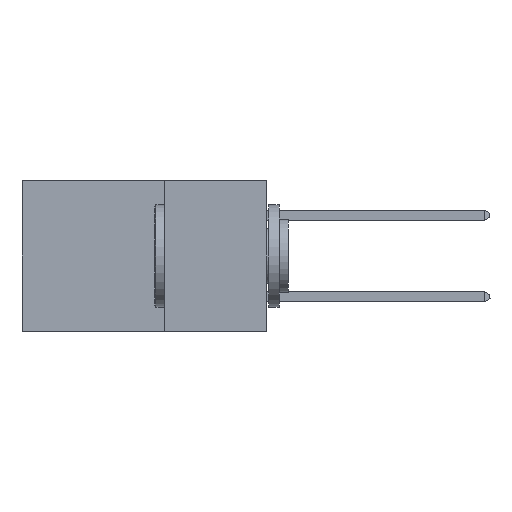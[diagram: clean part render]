
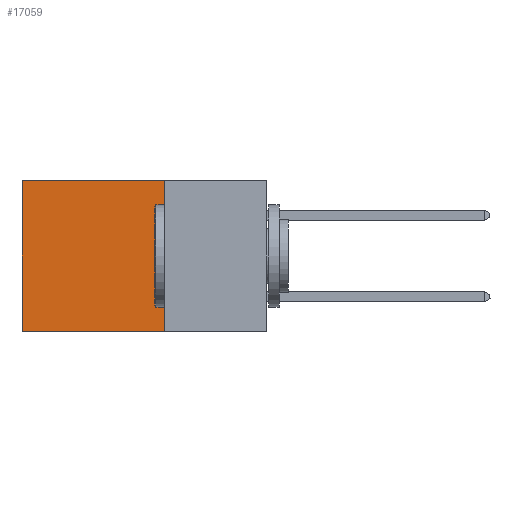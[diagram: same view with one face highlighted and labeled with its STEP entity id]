
A CAD part, left-side view. The second image highlights one B-rep face of the part: STEP entity #17059.
In plain terms, the highlighted planar face has unit normal (-1, 0, 0).
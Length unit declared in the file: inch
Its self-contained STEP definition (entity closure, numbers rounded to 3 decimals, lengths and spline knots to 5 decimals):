
#346 = VECTOR ( 'NONE', #17457, 39.37008 ) ;
#575 = DIRECTION ( 'NONE',  ( 0., 0., -1. ) ) ;
#2015 = LINE ( 'NONE', #3755, #9354 ) ;
#2084 = DIRECTION ( 'NONE',  ( 0., 1., 0. ) ) ;
#2139 = CARTESIAN_POINT ( 'NONE',  ( 0.2875, 0.6, 0. ) ) ;
#2925 = CARTESIAN_POINT ( 'NONE',  ( 0.2875, 0.6, 0. ) ) ;
#3717 = CARTESIAN_POINT ( 'NONE',  ( 0.2875, 0.25, 0. ) ) ;
#3755 = CARTESIAN_POINT ( 'NONE',  ( 0.2875, 0.25, 0. ) ) ;
#3989 = CARTESIAN_POINT ( 'NONE',  ( 0.2875, 0.25, -0.37 ) ) ;
#5107 = VERTEX_POINT ( 'NONE', #3989 ) ;
#5269 = CARTESIAN_POINT ( 'NONE',  ( 0.2875, 0.25, -0.37 ) ) ;
#5874 = ORIENTED_EDGE ( 'NONE', *, *, #10769, .F. ) ;
#6649 = ORIENTED_EDGE ( 'NONE', *, *, #21062, .T. ) ;
#6776 = AXIS2_PLACEMENT_3D ( 'NONE', #18778, #16770, #575 ) ;
#7679 = CARTESIAN_POINT ( 'NONE',  ( 0.2875, 0.25, 0. ) ) ;
#8809 = EDGE_CURVE ( 'NONE', #21136, #9579, #21199, .T. ) ;
#9354 = VECTOR ( 'NONE', #9521, 39.37008 ) ;
#9521 = DIRECTION ( 'NONE',  ( 0., 0., -1. ) ) ;
#9579 = VERTEX_POINT ( 'NONE', #13385 ) ;
#10769 = EDGE_CURVE ( 'NONE', #5107, #9579, #13221, .T. ) ;
#11998 = ORIENTED_EDGE ( 'NONE', *, *, #21715, .F. ) ;
#12818 = ORIENTED_EDGE ( 'NONE', *, *, #8809, .T. ) ;
#13094 = PLANE ( 'NONE',  #6776 ) ;
#13176 = EDGE_LOOP ( 'NONE', ( #12818, #5874, #11998, #6649 ) ) ;
#13221 = LINE ( 'NONE', #5269, #17226 ) ;
#13385 = CARTESIAN_POINT ( 'NONE',  ( 0.2875, 0.6, -0.37 ) ) ;
#13773 = FACE_OUTER_BOUND ( 'NONE', #13176, .T. ) ;
#16770 = DIRECTION ( 'NONE',  ( 1., 0., 0. ) ) ;
#17059 = ADVANCED_FACE ( 'NONE', ( #13773 ), #13094, .F. ) ;
#17226 = VECTOR ( 'NONE', #2084, 39.37008 ) ;
#17457 = DIRECTION ( 'NONE',  ( 0., 0., -1. ) ) ;
#18725 = VERTEX_POINT ( 'NONE', #7679 ) ;
#18778 = CARTESIAN_POINT ( 'NONE',  ( 0.2875, 0.25, 0. ) ) ;
#19922 = DIRECTION ( 'NONE',  ( 0., 1., 0. ) ) ;
#21062 = EDGE_CURVE ( 'NONE', #18725, #21136, #21713, .T. ) ;
#21136 = VERTEX_POINT ( 'NONE', #2139 ) ;
#21199 = LINE ( 'NONE', #2925, #346 ) ;
#21713 = LINE ( 'NONE', #3717, #21982 ) ;
#21715 = EDGE_CURVE ( 'NONE', #18725, #5107, #2015, .T. ) ;
#21982 = VECTOR ( 'NONE', #19922, 39.37008 ) ;
